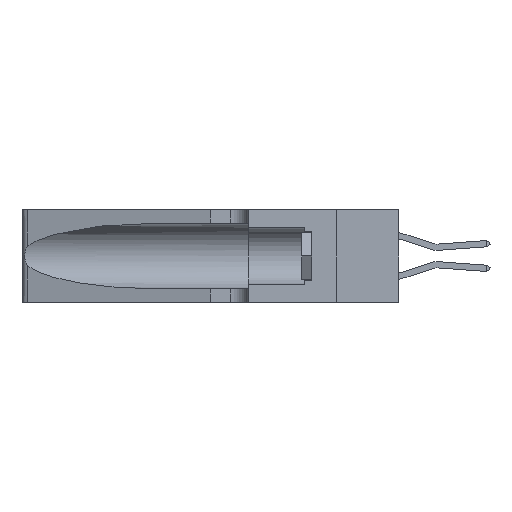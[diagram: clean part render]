
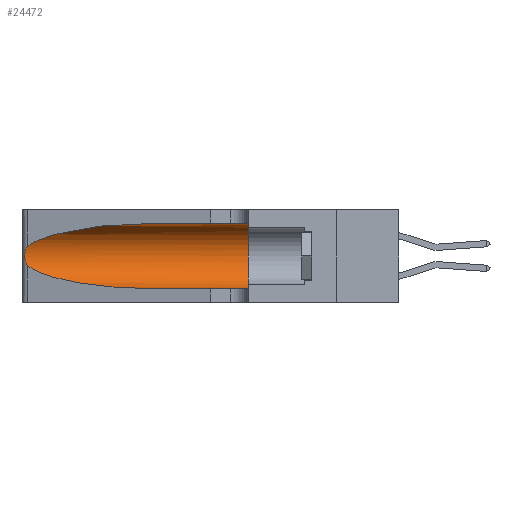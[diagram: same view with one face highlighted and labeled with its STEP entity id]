
A CAD part, left-side view. The second image highlights one B-rep face of the part: STEP entity #24472.
In plain terms, the highlighted cylindrical face has radius 3.308 mm (diameter 6.617 mm), a partial arc.
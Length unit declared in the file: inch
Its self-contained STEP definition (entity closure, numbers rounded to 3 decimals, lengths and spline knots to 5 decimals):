
#307 = VERTEX_POINT ( 'NONE', #5766 ) ;
#966 = CARTESIAN_POINT ( 'NONE',  ( 0.1305, 0.72297, 0.31525 ) ) ;
#1567 = CARTESIAN_POINT ( 'NONE',  ( 0.1305, 1.61858, 0.185 ) ) ;
#1832 = DIRECTION ( 'NONE',  ( 0., -1., 0. ) ) ;
#5478 = CARTESIAN_POINT ( 'NONE',  ( 0.25555, 1.22994, 0.2215 ) ) ;
#5538 =( BOUNDED_CURVE ( )  B_SPLINE_CURVE ( 3, ( #16881, #13785, #16517, #19485 ),
 .UNSPECIFIED., .F., .F. ) 
 B_SPLINE_CURVE_WITH_KNOTS ( ( 4, 4 ),
 ( 1.5708, 2.84003 ),
 .UNSPECIFIED. ) 
 CURVE ( )  GEOMETRIC_REPRESENTATION_ITEM ( )  RATIONAL_B_SPLINE_CURVE ( ( 1., 0.87, 0.87, 1. ) ) 
 REPRESENTATION_ITEM ( '' )  );
#5766 = CARTESIAN_POINT ( 'NONE',  ( 0.25487, 1.22718, 0.22369 ) ) ;
#6634 = LINE ( 'NONE', #13198, #10373 ) ;
#6688 = VERTEX_POINT ( 'NONE', #28686 ) ;
#6811 = ORIENTED_EDGE ( 'NONE', *, *, #36922, .T. ) ;
#7985 = AXIS2_PLACEMENT_3D ( 'NONE', #1567, #1832, #22599 ) ;
#8196 = CARTESIAN_POINT ( 'NONE',  ( 0.26018, 1.23835, 0.19895 ) ) ;
#8800 = EDGE_CURVE ( 'NONE', #36262, #24762, #9326, .T. ) ;
#9326 =( BOUNDED_CURVE ( )  B_SPLINE_CURVE ( 3, ( #31803, #11248, #20196, #23190 ),
 .UNSPECIFIED., .F., .F. ) 
 B_SPLINE_CURVE_WITH_KNOTS ( ( 4, 4 ),
 ( 3.44316, 4.71239 ),
 .UNSPECIFIED. ) 
 CURVE ( )  GEOMETRIC_REPRESENTATION_ITEM ( )  RATIONAL_B_SPLINE_CURVE ( ( 1., 0.87, 0.87, 1. ) ) 
 REPRESENTATION_ITEM ( '' )  );
#10373 = VECTOR ( 'NONE', #24786, 39.37008 ) ;
#11248 = CARTESIAN_POINT ( 'NONE',  ( 0.2373, 1.15595, 0.08982 ) ) ;
#11448 = VERTEX_POINT ( 'NONE', #26769 ) ;
#12216 = CARTESIAN_POINT ( 'NONE',  ( 0.1305, 1.61858, 0.05475 ) ) ;
#13069 = FACE_OUTER_BOUND ( 'NONE', #21915, .T. ) ;
#13198 = CARTESIAN_POINT ( 'NONE',  ( 0.1305, 1.61858, 0.31525 ) ) ;
#13785 = CARTESIAN_POINT ( 'NONE',  ( 0.18966, 0.96281, 0.31525 ) ) ;
#13971 = EDGE_CURVE ( 'NONE', #32591, #11448, #6634, .T. ) ;
#14334 = CARTESIAN_POINT ( 'NONE',  ( 0.25854, 1.2359, 0.20912 ) ) ;
#14922 = CYLINDRICAL_SURFACE ( 'NONE', #7985, 0.13025 ) ;
#15078 = B_SPLINE_CURVE_WITH_KNOTS ( 'NONE', 3,
 ( #25259, #5478, #25764, #22756, #14334, #8196, #19888, #35067, #37519, #34795, #28777, #19758, #29155, #22883 ),
 .UNSPECIFIED., .F., .F.,
 ( 4, 2, 2, 2, 2, 2, 4 ),
 ( 0., 0.00027, 0.00053, 0.00107, 0.0016, 0.00187, 0.00214 ),
 .UNSPECIFIED. ) ;
#15402 = LINE ( 'NONE', #12216, #15857 ) ;
#15736 = DIRECTION ( 'NONE',  ( 0., -1., 0. ) ) ;
#15857 = VECTOR ( 'NONE', #15736, 39.37008 ) ;
#16517 = CARTESIAN_POINT ( 'NONE',  ( 0.2373, 1.15595, 0.28018 ) ) ;
#16881 = CARTESIAN_POINT ( 'NONE',  ( 0.1305, 0.72297, 0.31525 ) ) ;
#17262 = DIRECTION ( 'NONE',  ( 0., 1., 0. ) ) ;
#17393 = CARTESIAN_POINT ( 'NONE',  ( 0.1305, 0.35, 0.185 ) ) ;
#19485 = CARTESIAN_POINT ( 'NONE',  ( 0.25487, 1.22718, 0.22369 ) ) ;
#19758 = CARTESIAN_POINT ( 'NONE',  ( 0.25639, 1.23186, 0.15144 ) ) ;
#19888 = CARTESIAN_POINT ( 'NONE',  ( 0.26075, 1.23896, 0.19203 ) ) ;
#19918 = ORIENTED_EDGE ( 'NONE', *, *, #28404, .F. ) ;
#20196 = CARTESIAN_POINT ( 'NONE',  ( 0.18966, 0.96281, 0.05475 ) ) ;
#21156 = CIRCLE ( 'NONE', #32255, 0.13025 ) ;
#21915 = EDGE_LOOP ( 'NONE', ( #6811, #31391, #27278, #26421, #19918, #35260 ) ) ;
#22365 = EDGE_CURVE ( 'NONE', #24762, #6688, #15402, .T. ) ;
#22599 = DIRECTION ( 'NONE',  ( 0., 0., -1. ) ) ;
#22756 = CARTESIAN_POINT ( 'NONE',  ( 0.25787, 1.23484, 0.2124 ) ) ;
#22883 = CARTESIAN_POINT ( 'NONE',  ( 0.25487, 1.22718, 0.14631 ) ) ;
#23190 = CARTESIAN_POINT ( 'NONE',  ( 0.1305, 0.72297, 0.05475 ) ) ;
#23943 = EDGE_CURVE ( 'NONE', #307, #36262, #15078, .T. ) ;
#24472 = ADVANCED_FACE ( 'NONE', ( #13069 ), #14922, .F. ) ;
#24762 = VERTEX_POINT ( 'NONE', #26624 ) ;
#24786 = DIRECTION ( 'NONE',  ( 0., -1., 0. ) ) ;
#25259 = CARTESIAN_POINT ( 'NONE',  ( 0.25487, 1.22718, 0.22369 ) ) ;
#25764 = CARTESIAN_POINT ( 'NONE',  ( 0.25639, 1.23184, 0.21858 ) ) ;
#26421 = ORIENTED_EDGE ( 'NONE', *, *, #22365, .T. ) ;
#26624 = CARTESIAN_POINT ( 'NONE',  ( 0.1305, 0.72297, 0.05475 ) ) ;
#26769 = CARTESIAN_POINT ( 'NONE',  ( 0.1305, 0.35, 0.31525 ) ) ;
#27278 = ORIENTED_EDGE ( 'NONE', *, *, #8800, .T. ) ;
#28404 = EDGE_CURVE ( 'NONE', #11448, #6688, #21156, .T. ) ;
#28686 = CARTESIAN_POINT ( 'NONE',  ( 0.1305, 0.35, 0.05475 ) ) ;
#28777 = CARTESIAN_POINT ( 'NONE',  ( 0.25789, 1.23486, 0.15765 ) ) ;
#29155 = CARTESIAN_POINT ( 'NONE',  ( 0.25555, 1.22993, 0.14849 ) ) ;
#30611 = CARTESIAN_POINT ( 'NONE',  ( 0.25487, 1.22718, 0.14631 ) ) ;
#31391 = ORIENTED_EDGE ( 'NONE', *, *, #23943, .T. ) ;
#31803 = CARTESIAN_POINT ( 'NONE',  ( 0.25487, 1.22718, 0.14631 ) ) ;
#32255 = AXIS2_PLACEMENT_3D ( 'NONE', #17393, #17262, #35288 ) ;
#32591 = VERTEX_POINT ( 'NONE', #966 ) ;
#34795 = CARTESIAN_POINT ( 'NONE',  ( 0.25856, 1.23593, 0.16098 ) ) ;
#35067 = CARTESIAN_POINT ( 'NONE',  ( 0.26075, 1.23896, 0.178 ) ) ;
#35260 = ORIENTED_EDGE ( 'NONE', *, *, #13971, .F. ) ;
#35288 = DIRECTION ( 'NONE',  ( 0., 0., 1. ) ) ;
#36262 = VERTEX_POINT ( 'NONE', #30611 ) ;
#36922 = EDGE_CURVE ( 'NONE', #32591, #307, #5538, .T. ) ;
#37519 = CARTESIAN_POINT ( 'NONE',  ( 0.26017, 1.23833, 0.17102 ) ) ;
